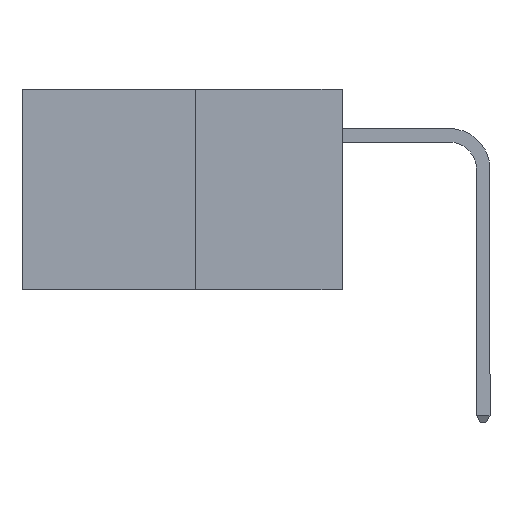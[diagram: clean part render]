
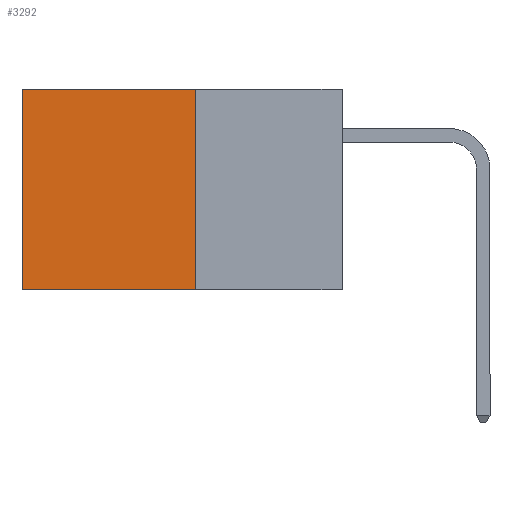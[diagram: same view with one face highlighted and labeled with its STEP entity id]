
A CAD part, left-side view. The second image highlights one B-rep face of the part: STEP entity #3292.
In plain terms, the highlighted planar face has unit normal (-1, 0, 0).
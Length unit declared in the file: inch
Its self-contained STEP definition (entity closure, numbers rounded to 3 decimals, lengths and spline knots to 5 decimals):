
#45 = VECTOR ( 'NONE', #4795, 39.37008 ) ;
#452 = AXIS2_PLACEMENT_3D ( 'NONE', #4695, #4664, #4633 ) ;
#550 = VECTOR ( 'NONE', #6474, 39.37008 ) ;
#812 = VERTEX_POINT ( 'NONE', #9827 ) ;
#957 = ORIENTED_EDGE ( 'NONE', *, *, #10505, .F. ) ;
#1854 = ORIENTED_EDGE ( 'NONE', *, *, #6190, .T. ) ;
#2268 = VECTOR ( 'NONE', #4887, 39.37008 ) ;
#2279 = VERTEX_POINT ( 'NONE', #10523 ) ;
#2362 = DIRECTION ( 'NONE',  ( 0., 0., -1. ) ) ;
#2400 = CARTESIAN_POINT ( 'NONE',  ( 0.277, 0.59, -0.37 ) ) ;
#3292 = ADVANCED_FACE ( 'NONE', ( #7078 ), #4722, .F. ) ;
#4035 = CARTESIAN_POINT ( 'NONE',  ( 0.277, 0.27, 0. ) ) ;
#4633 = DIRECTION ( 'NONE',  ( 0., 0., -1. ) ) ;
#4637 = ORIENTED_EDGE ( 'NONE', *, *, #7123, .F. ) ;
#4664 = DIRECTION ( 'NONE',  ( 1., 0., 0. ) ) ;
#4695 = CARTESIAN_POINT ( 'NONE',  ( 0.277, 0.27, -0.37 ) ) ;
#4722 = PLANE ( 'NONE',  #452 ) ;
#4795 = DIRECTION ( 'NONE',  ( 0., 1., 0. ) ) ;
#4887 = DIRECTION ( 'NONE',  ( 0., 1., 0. ) ) ;
#4921 = CARTESIAN_POINT ( 'NONE',  ( 0.277, 0.27, 0. ) ) ;
#5599 = VERTEX_POINT ( 'NONE', #5642 ) ;
#5642 = CARTESIAN_POINT ( 'NONE',  ( 0.277, 0.59, 0. ) ) ;
#6190 = EDGE_CURVE ( 'NONE', #5599, #2279, #10270, .T. ) ;
#6395 = EDGE_LOOP ( 'NONE', ( #1854, #4637, #957, #10690 ) ) ;
#6474 = DIRECTION ( 'NONE',  ( 0., 0., -1. ) ) ;
#7078 = FACE_OUTER_BOUND ( 'NONE', #6395, .T. ) ;
#7123 = EDGE_CURVE ( 'NONE', #812, #2279, #10590, .T. ) ;
#7266 = LINE ( 'NONE', #10465, #550 ) ;
#8161 = VECTOR ( 'NONE', #2362, 39.37008 ) ;
#8775 = LINE ( 'NONE', #4035, #2268 ) ;
#9648 = CARTESIAN_POINT ( 'NONE',  ( 0.277, 0.27, -0.37 ) ) ;
#9827 = CARTESIAN_POINT ( 'NONE',  ( 0.277, 0.27, -0.37 ) ) ;
#9910 = EDGE_CURVE ( 'NONE', #9930, #5599, #8775, .T. ) ;
#9930 = VERTEX_POINT ( 'NONE', #4921 ) ;
#10270 = LINE ( 'NONE', #2400, #8161 ) ;
#10465 = CARTESIAN_POINT ( 'NONE',  ( 0.277, 0.27, -0.37 ) ) ;
#10505 = EDGE_CURVE ( 'NONE', #9930, #812, #7266, .T. ) ;
#10523 = CARTESIAN_POINT ( 'NONE',  ( 0.277, 0.59, -0.37 ) ) ;
#10590 = LINE ( 'NONE', #9648, #45 ) ;
#10690 = ORIENTED_EDGE ( 'NONE', *, *, #9910, .T. ) ;
